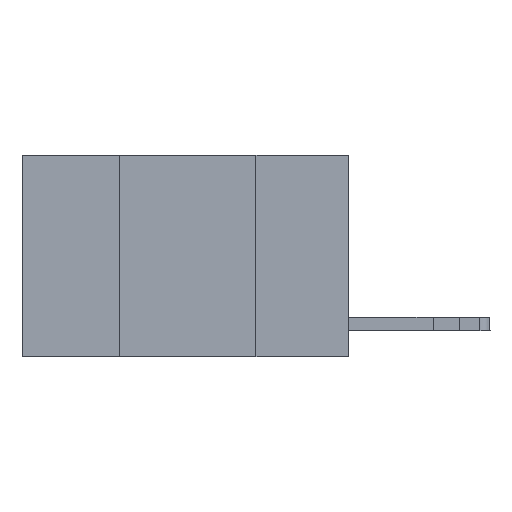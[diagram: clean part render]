
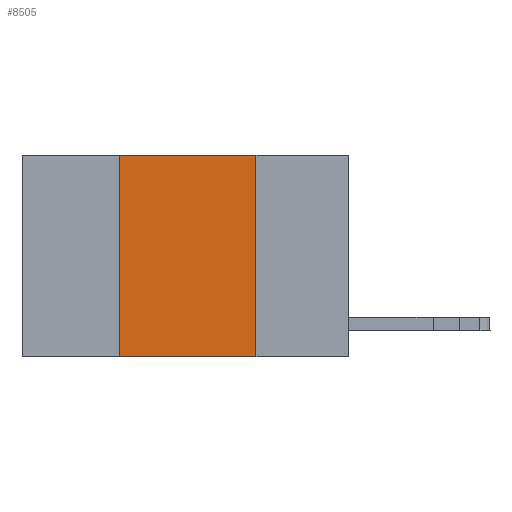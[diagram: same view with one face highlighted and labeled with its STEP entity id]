
A CAD part, left-side view. The second image highlights one B-rep face of the part: STEP entity #8505.
In plain terms, the highlighted planar face has unit normal (-1, 0, 0).
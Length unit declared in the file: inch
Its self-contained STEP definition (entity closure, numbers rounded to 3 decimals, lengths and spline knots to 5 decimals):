
#216 = EDGE_CURVE ( 'NONE', #2960, #15487, #11369, .T. ) ;
#1674 = CARTESIAN_POINT ( 'NONE',  ( 0., 0.42, 0. ) ) ;
#2656 = DIRECTION ( 'NONE',  ( 0., -1., 0. ) ) ;
#2815 = DIRECTION ( 'NONE',  ( 0., -1., 0. ) ) ;
#2935 = CARTESIAN_POINT ( 'NONE',  ( 0., 0.17, -0.37 ) ) ;
#2960 = VERTEX_POINT ( 'NONE', #24759 ) ;
#3761 = ORIENTED_EDGE ( 'NONE', *, *, #11053, .F. ) ;
#3825 = ORIENTED_EDGE ( 'NONE', *, *, #216, .T. ) ;
#6136 = EDGE_CURVE ( 'NONE', #2960, #10691, #7887, .T. ) ;
#7230 = CARTESIAN_POINT ( 'NONE',  ( 0., 0.6, 0. ) ) ;
#7887 = LINE ( 'NONE', #1674, #14471 ) ;
#8335 = EDGE_CURVE ( 'NONE', #26327, #15487, #10931, .T. ) ;
#8505 = ADVANCED_FACE ( 'NONE', ( #13831 ), #18252, .F. ) ;
#8747 = VECTOR ( 'NONE', #2656, 39.37008 ) ;
#10691 = VERTEX_POINT ( 'NONE', #18055 ) ;
#10931 = LINE ( 'NONE', #15507, #26361 ) ;
#10999 = CARTESIAN_POINT ( 'NONE',  ( 0., 0.17, 0. ) ) ;
#11053 = EDGE_CURVE ( 'NONE', #10691, #26327, #26196, .T. ) ;
#11369 = LINE ( 'NONE', #17611, #8747 ) ;
#13690 = DIRECTION ( 'NONE',  ( 0., 0., -1. ) ) ;
#13831 = FACE_OUTER_BOUND ( 'NONE', #20487, .T. ) ;
#14005 = AXIS2_PLACEMENT_3D ( 'NONE', #24075, #22265, #13690 ) ;
#14471 = VECTOR ( 'NONE', #16347, 39.37008 ) ;
#15487 = VERTEX_POINT ( 'NONE', #2935 ) ;
#15507 = CARTESIAN_POINT ( 'NONE',  ( 0., 0.17, 0. ) ) ;
#16347 = DIRECTION ( 'NONE',  ( 0., 0., 1. ) ) ;
#17611 = CARTESIAN_POINT ( 'NONE',  ( 0., 0.6, -0.37 ) ) ;
#18055 = CARTESIAN_POINT ( 'NONE',  ( 0., 0.42, 0. ) ) ;
#18056 = ORIENTED_EDGE ( 'NONE', *, *, #6136, .F. ) ;
#18252 = PLANE ( 'NONE',  #14005 ) ;
#19365 = VECTOR ( 'NONE', #2815, 39.37008 ) ;
#20487 = EDGE_LOOP ( 'NONE', ( #24833, #3761, #18056, #3825 ) ) ;
#22265 = DIRECTION ( 'NONE',  ( 1., 0., 0. ) ) ;
#24075 = CARTESIAN_POINT ( 'NONE',  ( 0., 0.6, 0. ) ) ;
#24759 = CARTESIAN_POINT ( 'NONE',  ( 0., 0.42, -0.37 ) ) ;
#24833 = ORIENTED_EDGE ( 'NONE', *, *, #8335, .F. ) ;
#25862 = DIRECTION ( 'NONE',  ( 0., 0., -1. ) ) ;
#26196 = LINE ( 'NONE', #7230, #19365 ) ;
#26327 = VERTEX_POINT ( 'NONE', #10999 ) ;
#26361 = VECTOR ( 'NONE', #25862, 39.37008 ) ;
